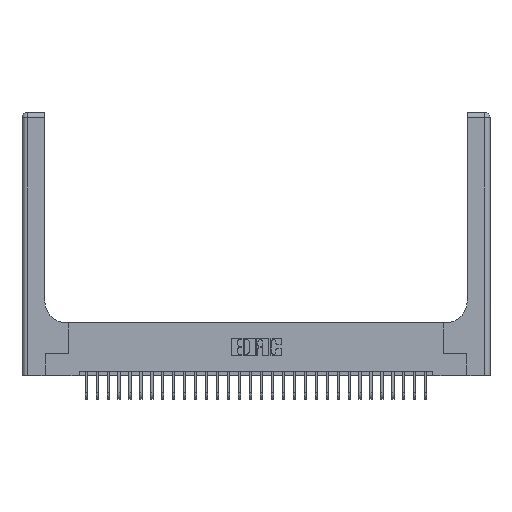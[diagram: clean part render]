
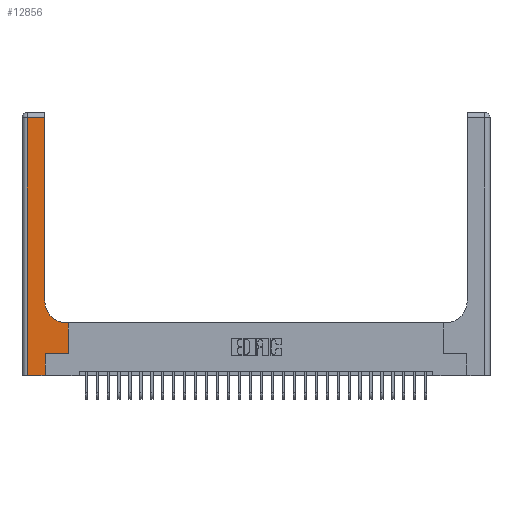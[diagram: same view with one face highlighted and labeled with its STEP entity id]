
A CAD part, top view. The second image highlights one B-rep face of the part: STEP entity #12856.
In plain terms, the highlighted planar face has unit normal (0, 0, 1).
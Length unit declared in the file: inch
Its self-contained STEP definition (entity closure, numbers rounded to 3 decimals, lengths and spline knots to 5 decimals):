
#15 = LINE ( 'NONE', #13072, #20200 ) ;
#970 = VERTEX_POINT ( 'NONE', #9903 ) ;
#1356 = LINE ( 'NONE', #2359, #12009 ) ;
#1479 = CIRCLE ( 'NONE', #26819, 0.25 ) ;
#1505 = ORIENTED_EDGE ( 'NONE', *, *, #10272, .T. ) ;
#2359 = CARTESIAN_POINT ( 'NONE',  ( 0., 0., 0.37 ) ) ;
#3111 = DIRECTION ( 'NONE',  ( -1., 0., 0. ) ) ;
#3393 = ORIENTED_EDGE ( 'NONE', *, *, #11331, .T. ) ;
#3778 = LINE ( 'NONE', #4274, #12954 ) ;
#4274 = CARTESIAN_POINT ( 'NONE',  ( 0.528, 0.25, 0.37 ) ) ;
#4377 = DIRECTION ( 'NONE',  ( -1., 0., 0. ) ) ;
#4409 = ORIENTED_EDGE ( 'NONE', *, *, #5931, .T. ) ;
#4550 = ORIENTED_EDGE ( 'NONE', *, *, #21824, .T. ) ;
#4617 = VECTOR ( 'NONE', #26725, 39.37008 ) ;
#4819 = DIRECTION ( 'NONE',  ( 1., 0., 0. ) ) ;
#5022 = CARTESIAN_POINT ( 'NONE',  ( 0.528, 0.6, 0.37 ) ) ;
#5367 = DIRECTION ( 'NONE',  ( 0., 1., 0. ) ) ;
#5629 = ORIENTED_EDGE ( 'NONE', *, *, #25143, .T. ) ;
#5931 = EDGE_CURVE ( 'NONE', #10937, #17386, #25620, .T. ) ;
#6777 = CARTESIAN_POINT ( 'NONE',  ( 0.26, 0.6, 0.37 ) ) ;
#7199 = VECTOR ( 'NONE', #4819, 39.37008 ) ;
#7488 = CARTESIAN_POINT ( 'NONE',  ( 0.06, 2.94, 0.37 ) ) ;
#7666 = CARTESIAN_POINT ( 'NONE',  ( 0.51, 0.6, 0.37 ) ) ;
#8413 = EDGE_CURVE ( 'NONE', #12917, #10937, #1479, .T. ) ;
#8586 = DIRECTION ( 'NONE',  ( 1., 0., 0. ) ) ;
#8646 = FACE_OUTER_BOUND ( 'NONE', #26051, .T. ) ;
#8878 = CARTESIAN_POINT ( 'NONE',  ( 0.26, 0.85, 0.37 ) ) ;
#9419 = DIRECTION ( 'NONE',  ( 0., 0., -1. ) ) ;
#9903 = CARTESIAN_POINT ( 'NONE',  ( 0.06, 0., 0.37 ) ) ;
#10272 = EDGE_CURVE ( 'NONE', #970, #23181, #1356, .T. ) ;
#10325 = DIRECTION ( 'NONE',  ( 0., 1., 0. ) ) ;
#10937 = VERTEX_POINT ( 'NONE', #8878 ) ;
#11137 = VERTEX_POINT ( 'NONE', #7488 ) ;
#11331 = EDGE_CURVE ( 'NONE', #23181, #14374, #15811, .T. ) ;
#11883 = AXIS2_PLACEMENT_3D ( 'NONE', #18296, #9419, #3111 ) ;
#12009 = VECTOR ( 'NONE', #8586, 39.37008 ) ;
#12093 = CARTESIAN_POINT ( 'NONE',  ( 0.26, 3., 0.37 ) ) ;
#12856 = ADVANCED_FACE ( 'NONE', ( #8646 ), #27296, .F. ) ;
#12878 = LINE ( 'NONE', #16155, #7199 ) ;
#12917 = VERTEX_POINT ( 'NONE', #7666 ) ;
#12932 = CARTESIAN_POINT ( 'NONE',  ( 0.51, 0.85, 0.37 ) ) ;
#12954 = VECTOR ( 'NONE', #29005, 39.37008 ) ;
#13072 = CARTESIAN_POINT ( 'NONE',  ( 0.06, 3., 0.37 ) ) ;
#13295 = ORIENTED_EDGE ( 'NONE', *, *, #8413, .T. ) ;
#13622 = CARTESIAN_POINT ( 'NONE',  ( 0.528, 0.25, 0.37 ) ) ;
#14374 = VERTEX_POINT ( 'NONE', #14974 ) ;
#14974 = CARTESIAN_POINT ( 'NONE',  ( 0.265, 0.25, 0.37 ) ) ;
#15811 = LINE ( 'NONE', #25861, #17588 ) ;
#16109 = VECTOR ( 'NONE', #4377, 39.37008 ) ;
#16155 = CARTESIAN_POINT ( 'NONE',  ( 0.265, 0.25, 0.37 ) ) ;
#16833 = LINE ( 'NONE', #22561, #16109 ) ;
#17168 = DIRECTION ( 'NONE',  ( 0., 0., -1. ) ) ;
#17386 = VERTEX_POINT ( 'NONE', #26581 ) ;
#17519 = VERTEX_POINT ( 'NONE', #13622 ) ;
#17588 = VECTOR ( 'NONE', #10325, 39.37008 ) ;
#17592 = VERTEX_POINT ( 'NONE', #5022 ) ;
#18296 = CARTESIAN_POINT ( 'NONE',  ( 0., 3., 0.37 ) ) ;
#18628 = EDGE_CURVE ( 'NONE', #11137, #970, #15, .T. ) ;
#18700 = ORIENTED_EDGE ( 'NONE', *, *, #18628, .T. ) ;
#19668 = VECTOR ( 'NONE', #5367, 39.37008 ) ;
#19935 = EDGE_CURVE ( 'NONE', #14374, #17519, #12878, .T. ) ;
#20200 = VECTOR ( 'NONE', #28711, 39.37008 ) ;
#21824 = EDGE_CURVE ( 'NONE', #17592, #12917, #26794, .T. ) ;
#22506 = CARTESIAN_POINT ( 'NONE',  ( 0.265, 0., 0.37 ) ) ;
#22561 = CARTESIAN_POINT ( 'NONE',  ( 0., 2.94, 0.37 ) ) ;
#22713 = ORIENTED_EDGE ( 'NONE', *, *, #25094, .T. ) ;
#23181 = VERTEX_POINT ( 'NONE', #22506 ) ;
#25094 = EDGE_CURVE ( 'NONE', #17386, #11137, #16833, .T. ) ;
#25143 = EDGE_CURVE ( 'NONE', #17519, #17592, #3778, .T. ) ;
#25620 = LINE ( 'NONE', #12093, #19668 ) ;
#25861 = CARTESIAN_POINT ( 'NONE',  ( 0.265, 0., 0.37 ) ) ;
#25966 = ORIENTED_EDGE ( 'NONE', *, *, #19935, .T. ) ;
#26051 = EDGE_LOOP ( 'NONE', ( #4409, #22713, #18700, #1505, #3393, #25966, #5629, #4550, #13295 ) ) ;
#26581 = CARTESIAN_POINT ( 'NONE',  ( 0.26, 2.94, 0.37 ) ) ;
#26725 = DIRECTION ( 'NONE',  ( -1., 0., 0. ) ) ;
#26794 = LINE ( 'NONE', #6777, #4617 ) ;
#26819 = AXIS2_PLACEMENT_3D ( 'NONE', #12932, #17168, #28366 ) ;
#27296 = PLANE ( 'NONE',  #11883 ) ;
#28366 = DIRECTION ( 'NONE',  ( 1., 0., 0. ) ) ;
#28711 = DIRECTION ( 'NONE',  ( 0., -1., 0. ) ) ;
#29005 = DIRECTION ( 'NONE',  ( 0., 1., 0. ) ) ;
